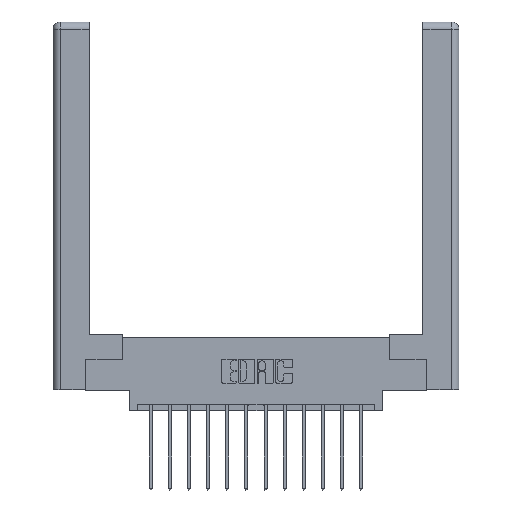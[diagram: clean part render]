
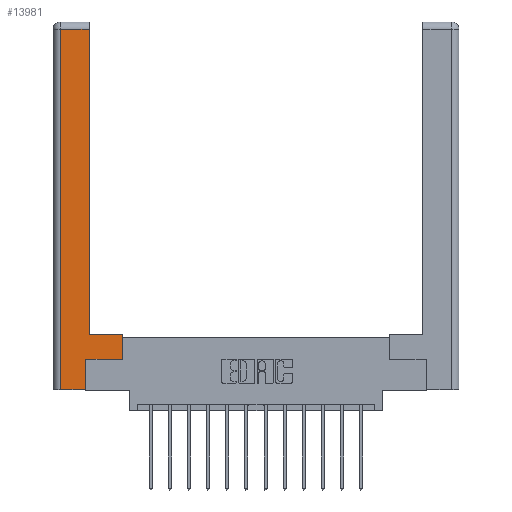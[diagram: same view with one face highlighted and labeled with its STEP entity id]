
A CAD part, top view. The second image highlights one B-rep face of the part: STEP entity #13981.
In plain terms, the highlighted planar face has unit normal (0, 0, 1).
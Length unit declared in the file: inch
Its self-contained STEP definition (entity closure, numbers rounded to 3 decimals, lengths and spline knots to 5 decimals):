
#265 = EDGE_CURVE ( 'NONE', #4852, #5776, #3096, .T. ) ;
#938 = VECTOR ( 'NONE', #9196, 39.37008 ) ;
#1010 = ORIENTED_EDGE ( 'NONE', *, *, #10337, .T. ) ;
#1103 = CARTESIAN_POINT ( 'NONE',  ( 0.265, 0., 0. ) ) ;
#1168 = CARTESIAN_POINT ( 'NONE',  ( 0.295, 3., 0. ) ) ;
#1371 = VERTEX_POINT ( 'NONE', #4316 ) ;
#1418 = VERTEX_POINT ( 'NONE', #1734 ) ;
#1456 = VERTEX_POINT ( 'NONE', #11875 ) ;
#1734 = CARTESIAN_POINT ( 'NONE',  ( 0.295, 0.45, 0. ) ) ;
#2316 = ORIENTED_EDGE ( 'NONE', *, *, #265, .T. ) ;
#2668 = DIRECTION ( 'NONE',  ( -1., 0., 0. ) ) ;
#2908 = EDGE_LOOP ( 'NONE', ( #11723, #7428, #10531, #15540, #5244, #2316, #11669, #1010 ) ) ;
#2960 = DIRECTION ( 'NONE',  ( 0., -1., 0. ) ) ;
#3096 = LINE ( 'NONE', #5299, #10069 ) ;
#3130 = CARTESIAN_POINT ( 'NONE',  ( 0.565, 0.45, 0. ) ) ;
#3870 = DIRECTION ( 'NONE',  ( 1., 0., 0. ) ) ;
#4101 = LINE ( 'NONE', #12607, #13783 ) ;
#4102 = EDGE_CURVE ( 'NONE', #1371, #11147, #7332, .T. ) ;
#4316 = CARTESIAN_POINT ( 'NONE',  ( 0.0615, 0., 0. ) ) ;
#4601 = VECTOR ( 'NONE', #8640, 39.37008 ) ;
#4669 = FACE_OUTER_BOUND ( 'NONE', #2908, .T. ) ;
#4852 = VERTEX_POINT ( 'NONE', #13585 ) ;
#5244 = ORIENTED_EDGE ( 'NONE', *, *, #5622, .T. ) ;
#5299 = CARTESIAN_POINT ( 'NONE',  ( 0.565, 0.245, 0. ) ) ;
#5474 = AXIS2_PLACEMENT_3D ( 'NONE', #11920, #12171, #13186 ) ;
#5603 = LINE ( 'NONE', #1168, #4601 ) ;
#5622 = EDGE_CURVE ( 'NONE', #11147, #4852, #14078, .T. ) ;
#5638 = LINE ( 'NONE', #11547, #938 ) ;
#5776 = VERTEX_POINT ( 'NONE', #11473 ) ;
#6348 = EDGE_CURVE ( 'NONE', #15535, #1371, #9792, .T. ) ;
#6438 = DIRECTION ( 'NONE',  ( 0., 1., 0. ) ) ;
#6570 = VECTOR ( 'NONE', #2960, 39.37008 ) ;
#7332 = LINE ( 'NONE', #8758, #8241 ) ;
#7428 = ORIENTED_EDGE ( 'NONE', *, *, #13871, .T. ) ;
#8241 = VECTOR ( 'NONE', #12297, 39.37008 ) ;
#8322 = VECTOR ( 'NONE', #12979, 39.37008 ) ;
#8500 = VECTOR ( 'NONE', #6438, 39.37008 ) ;
#8640 = DIRECTION ( 'NONE',  ( 0., 1., 0. ) ) ;
#8758 = CARTESIAN_POINT ( 'NONE',  ( 0.265, 0., 0. ) ) ;
#9196 = DIRECTION ( 'NONE',  ( -1., 0., 0. ) ) ;
#9262 = CARTESIAN_POINT ( 'NONE',  ( 0.0615, 0., 0. ) ) ;
#9792 = LINE ( 'NONE', #9262, #6570 ) ;
#10069 = VECTOR ( 'NONE', #3870, 39.37008 ) ;
#10337 = EDGE_CURVE ( 'NONE', #1456, #1418, #5638, .T. ) ;
#10531 = ORIENTED_EDGE ( 'NONE', *, *, #6348, .T. ) ;
#11147 = VERTEX_POINT ( 'NONE', #1103 ) ;
#11473 = CARTESIAN_POINT ( 'NONE',  ( 0.565, 0.245, 0. ) ) ;
#11547 = CARTESIAN_POINT ( 'NONE',  ( 0.295, 0.45, 0. ) ) ;
#11591 = CARTESIAN_POINT ( 'NONE',  ( 0.265, 0.245, 0. ) ) ;
#11669 = ORIENTED_EDGE ( 'NONE', *, *, #14429, .T. ) ;
#11723 = ORIENTED_EDGE ( 'NONE', *, *, #15676, .T. ) ;
#11860 = VERTEX_POINT ( 'NONE', #12989 ) ;
#11875 = CARTESIAN_POINT ( 'NONE',  ( 0.565, 0.45, 0. ) ) ;
#11920 = CARTESIAN_POINT ( 'NONE',  ( 0., 0., 0. ) ) ;
#12171 = DIRECTION ( 'NONE',  ( 0., 0., -1. ) ) ;
#12297 = DIRECTION ( 'NONE',  ( 1., 0., 0. ) ) ;
#12607 = CARTESIAN_POINT ( 'NONE',  ( 0.0615, 2.94, 0. ) ) ;
#12979 = DIRECTION ( 'NONE',  ( 0., 1., 0. ) ) ;
#12989 = CARTESIAN_POINT ( 'NONE',  ( 0.295, 2.94, 0. ) ) ;
#13186 = DIRECTION ( 'NONE',  ( -1., 0., 0. ) ) ;
#13585 = CARTESIAN_POINT ( 'NONE',  ( 0.265, 0.245, 0. ) ) ;
#13783 = VECTOR ( 'NONE', #2668, 39.37008 ) ;
#13871 = EDGE_CURVE ( 'NONE', #11860, #15535, #4101, .T. ) ;
#13981 = ADVANCED_FACE ( 'NONE', ( #4669 ), #15212, .F. ) ;
#14078 = LINE ( 'NONE', #11591, #8500 ) ;
#14429 = EDGE_CURVE ( 'NONE', #5776, #1456, #15324, .T. ) ;
#14489 = CARTESIAN_POINT ( 'NONE',  ( 0.0615, 2.94, 0. ) ) ;
#15212 = PLANE ( 'NONE',  #5474 ) ;
#15324 = LINE ( 'NONE', #3130, #8322 ) ;
#15535 = VERTEX_POINT ( 'NONE', #14489 ) ;
#15540 = ORIENTED_EDGE ( 'NONE', *, *, #4102, .T. ) ;
#15676 = EDGE_CURVE ( 'NONE', #1418, #11860, #5603, .T. ) ;
